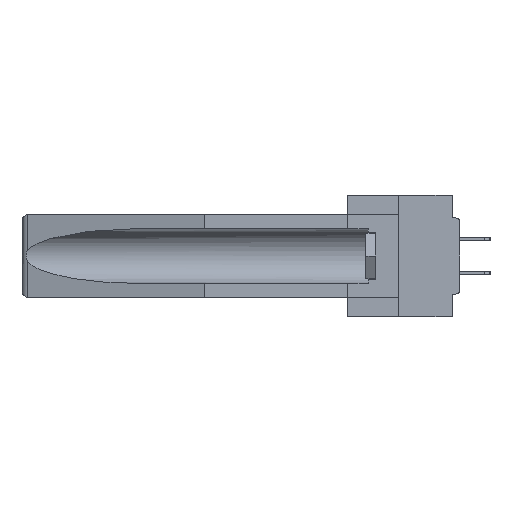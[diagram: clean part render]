
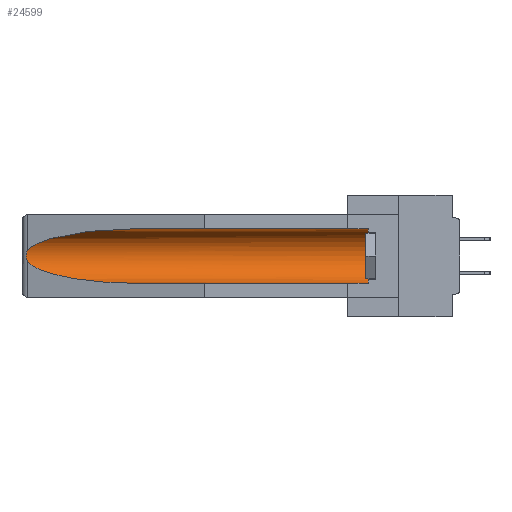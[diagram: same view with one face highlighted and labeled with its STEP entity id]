
A CAD part, left-side view. The second image highlights one B-rep face of the part: STEP entity #24599.
In plain terms, the highlighted cylindrical face has radius 2.857 mm (diameter 5.715 mm), a partial arc.
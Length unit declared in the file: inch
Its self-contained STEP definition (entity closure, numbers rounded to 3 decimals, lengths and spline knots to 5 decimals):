
#1126 = CARTESIAN_POINT ( 'NONE',  ( 0.26537, 1.52718, -0.14972 ) ) ;
#1475 = CARTESIAN_POINT ( 'NONE',  ( 0.26537, 1.52718, -0.19328 ) ) ;
#1774 = CARTESIAN_POINT ( 'NONE',  ( 0.155, 1.07973, -0.284 ) ) ;
#1935 = CARTESIAN_POINT ( 'NONE',  ( 0.21114, 1.30732, -0.284 ) ) ;
#2188 = VERTEX_POINT ( 'NONE', #29586 ) ;
#3547 = CARTESIAN_POINT ( 'NONE',  ( 0.155, -0.30754, -0.059 ) ) ;
#4252 = ORIENTED_EDGE ( 'NONE', *, *, #28374, .T. ) ;
#4512 = CARTESIAN_POINT ( 'NONE',  ( 0.2673, 1.53269, -0.17917 ) ) ;
#4551 = CARTESIAN_POINT ( 'NONE',  ( 0.155, 1.07973, -0.059 ) ) ;
#6303 = VERTEX_POINT ( 'NONE', #24989 ) ;
#6326 = CARTESIAN_POINT ( 'NONE',  ( 0.155, 0.126, -0.059 ) ) ;
#6614 = ORIENTED_EDGE ( 'NONE', *, *, #15300, .F. ) ;
#7063 = FACE_OUTER_BOUND ( 'NONE', #40605, .T. ) ;
#7599 = AXIS2_PLACEMENT_3D ( 'NONE', #24868, #25324, #22510 ) ;
#8103 = LINE ( 'NONE', #23507, #40439 ) ;
#8396 = CARTESIAN_POINT ( 'NONE',  ( 0.26597, 1.5296, -0.19026 ) ) ;
#8708 = EDGE_CURVE ( 'NONE', #15196, #23489, #37238, .T. ) ;
#9658 = ORIENTED_EDGE ( 'NONE', *, *, #43105, .T. ) ;
#9836 = DIRECTION ( 'NONE',  ( 0., 1., 0. ) ) ;
#10712 = LINE ( 'NONE', #3547, #24010 ) ;
#11239 = CARTESIAN_POINT ( 'NONE',  ( 0.2675, 1.53308, -0.16763 ) ) ;
#14376 = CARTESIAN_POINT ( 'NONE',  ( 0.26597, 1.52961, -0.15275 ) ) ;
#15079 = VERTEX_POINT ( 'NONE', #41137 ) ;
#15196 = VERTEX_POINT ( 'NONE', #28996 ) ;
#15216 = CARTESIAN_POINT ( 'NONE',  ( 0.26537, 1.52718, -0.14972 ) ) ;
#15300 = EDGE_CURVE ( 'NONE', #2188, #6303, #8103, .T. ) ;
#15447 = EDGE_CURVE ( 'NONE', #36841, #15196, #10712, .T. ) ;
#15663 = DIRECTION ( 'NONE',  ( 0., -1., 0. ) ) ;
#17780 = CIRCLE ( 'NONE', #20105, 0.1125 ) ;
#20105 = AXIS2_PLACEMENT_3D ( 'NONE', #22338, #15663, #32265 ) ;
#20629 = ORIENTED_EDGE ( 'NONE', *, *, #15447, .T. ) ;
#21174 = CARTESIAN_POINT ( 'NONE',  ( 0.2675, 1.53308, -0.17534 ) ) ;
#22338 = CARTESIAN_POINT ( 'NONE',  ( 0.155, 0.126, -0.1715 ) ) ;
#22510 = DIRECTION ( 'NONE',  ( 0., 0., 1. ) ) ;
#23489 = VERTEX_POINT ( 'NONE', #15216 ) ;
#23507 = CARTESIAN_POINT ( 'NONE',  ( 0.155, -0.30754, -0.284 ) ) ;
#24010 = VECTOR ( 'NONE', #28043, 39.37008 ) ;
#24599 = ADVANCED_FACE ( 'NONE', ( #7063 ), #41495, .F. ) ;
#24868 = CARTESIAN_POINT ( 'NONE',  ( 0.155, -0.30754, -0.1715 ) ) ;
#24989 = CARTESIAN_POINT ( 'NONE',  ( 0.155, 1.07973, -0.284 ) ) ;
#25324 = DIRECTION ( 'NONE',  ( 0., 1., 0. ) ) ;
#25345 = CARTESIAN_POINT ( 'NONE',  ( 0.26537, 1.52718, -0.19328 ) ) ;
#28043 = DIRECTION ( 'NONE',  ( 0., 1., 0. ) ) ;
#28134 = CARTESIAN_POINT ( 'NONE',  ( 0.2673, 1.5327, -0.16383 ) ) ;
#28374 = EDGE_CURVE ( 'NONE', #15079, #6303, #33465, .T. ) ;
#28543 = CARTESIAN_POINT ( 'NONE',  ( 0.25451, 1.48313, -0.24835 ) ) ;
#28996 = CARTESIAN_POINT ( 'NONE',  ( 0.155, 1.07973, -0.059 ) ) ;
#29586 = CARTESIAN_POINT ( 'NONE',  ( 0.155, 0.126, -0.284 ) ) ;
#32265 = DIRECTION ( 'NONE',  ( 0., 0., 1. ) ) ;
#33465 =( BOUNDED_CURVE ( )  B_SPLINE_CURVE ( 3, ( #1475, #28543, #1935, #1774 ),
 .UNSPECIFIED., .F., .F. ) 
 B_SPLINE_CURVE_WITH_KNOTS ( ( 4, 4 ),
 ( 0.1948, 1.5708 ),
 .UNSPECIFIED. ) 
 CURVE ( )  GEOMETRIC_REPRESENTATION_ITEM ( )  RATIONAL_B_SPLINE_CURVE ( ( 1., 0.848, 0.848, 1. ) ) 
 REPRESENTATION_ITEM ( '' )  );
#34946 = CARTESIAN_POINT ( 'NONE',  ( 0.26655, 1.53094, -0.18657 ) ) ;
#34986 = CARTESIAN_POINT ( 'NONE',  ( 0.21114, 1.30732, -0.059 ) ) ;
#35018 = ORIENTED_EDGE ( 'NONE', *, *, #8708, .T. ) ;
#35243 = CARTESIAN_POINT ( 'NONE',  ( 0.26537, 1.52718, -0.14972 ) ) ;
#36841 = VERTEX_POINT ( 'NONE', #6326 ) ;
#37238 =( BOUNDED_CURVE ( )  B_SPLINE_CURVE ( 3, ( #4551, #34986, #38400, #1126 ),
 .UNSPECIFIED., .F., .F. ) 
 B_SPLINE_CURVE_WITH_KNOTS ( ( 4, 4 ),
 ( 4.71239, 6.08839 ),
 .UNSPECIFIED. ) 
 CURVE ( )  GEOMETRIC_REPRESENTATION_ITEM ( )  RATIONAL_B_SPLINE_CURVE ( ( 1., 0.848, 0.848, 1. ) ) 
 REPRESENTATION_ITEM ( '' )  );
#38400 = CARTESIAN_POINT ( 'NONE',  ( 0.25451, 1.48313, -0.09465 ) ) ;
#38623 = B_SPLINE_CURVE_WITH_KNOTS ( 'NONE', 3,
 ( #35243, #14376, #41437, #28134, #11239, #21174, #4512, #34946, #8396, #25345 ),
 .UNSPECIFIED., .F., .F.,
 ( 4, 2, 2, 2, 4 ),
 ( 0., 0.00029, 0.00058, 0.00087, 0.00117 ),
 .UNSPECIFIED. ) ;
#39645 = EDGE_CURVE ( 'NONE', #23489, #15079, #38623, .T. ) ;
#39787 = ORIENTED_EDGE ( 'NONE', *, *, #39645, .T. ) ;
#40439 = VECTOR ( 'NONE', #9836, 39.37008 ) ;
#40605 = EDGE_LOOP ( 'NONE', ( #35018, #39787, #4252, #6614, #9658, #20629 ) ) ;
#41137 = CARTESIAN_POINT ( 'NONE',  ( 0.26537, 1.52718, -0.19328 ) ) ;
#41437 = CARTESIAN_POINT ( 'NONE',  ( 0.26654, 1.53092, -0.15636 ) ) ;
#41495 = CYLINDRICAL_SURFACE ( 'NONE', #7599, 0.1125 ) ;
#43105 = EDGE_CURVE ( 'NONE', #2188, #36841, #17780, .T. ) ;
